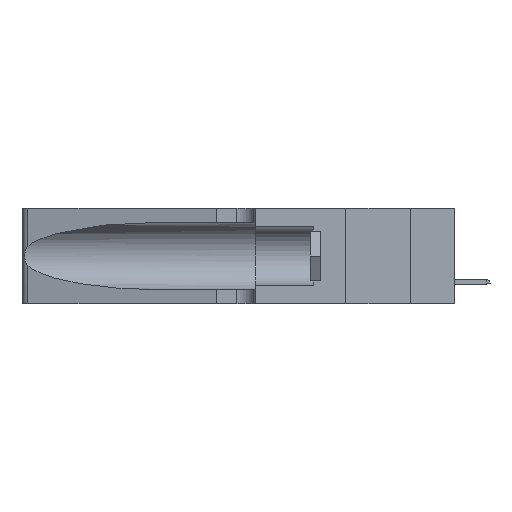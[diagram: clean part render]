
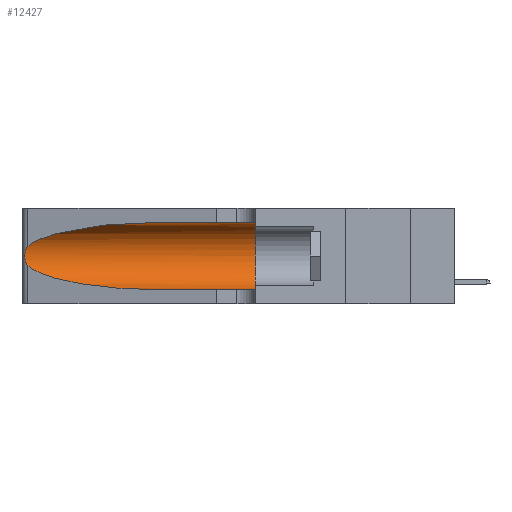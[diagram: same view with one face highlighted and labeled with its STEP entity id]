
A CAD part, left-side view. The second image highlights one B-rep face of the part: STEP entity #12427.
In plain terms, the highlighted cylindrical face has radius 3.308 mm (diameter 6.617 mm), a partial arc.
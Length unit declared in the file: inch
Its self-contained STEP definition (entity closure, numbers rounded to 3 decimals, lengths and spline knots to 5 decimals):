
#204 = CARTESIAN_POINT ( 'NONE',  ( 0.18966, 0.96281, 0.05475 ) ) ;
#894 = LINE ( 'NONE', #17572, #18752 ) ;
#1700 = EDGE_CURVE ( 'NONE', #21405, #21817, #20528, .T. ) ;
#2361 = CARTESIAN_POINT ( 'NONE',  ( 0.2373, 1.15595, 0.08982 ) ) ;
#3760 = CARTESIAN_POINT ( 'NONE',  ( 0.2373, 1.15595, 0.28018 ) ) ;
#3841 = CARTESIAN_POINT ( 'NONE',  ( 0.25787, 1.23484, 0.2124 ) ) ;
#4401 = CARTESIAN_POINT ( 'NONE',  ( 0.1305, 0.35, 0.185 ) ) ;
#4836 = ORIENTED_EDGE ( 'NONE', *, *, #15685, .T. ) ;
#4950 = FACE_OUTER_BOUND ( 'NONE', #5608, .T. ) ;
#5600 = CARTESIAN_POINT ( 'NONE',  ( 0.25854, 1.2359, 0.20912 ) ) ;
#5608 = EDGE_LOOP ( 'NONE', ( #13144, #4836, #24133, #20268, #17109, #25345 ) ) ;
#6421 = DIRECTION ( 'NONE',  ( 0., 1., 0. ) ) ;
#7059 = CARTESIAN_POINT ( 'NONE',  ( 0.1305, 0.35, 0.31525 ) ) ;
#7375 = EDGE_CURVE ( 'NONE', #21405, #19061, #19335, .T. ) ;
#7846 = CARTESIAN_POINT ( 'NONE',  ( 0.1305, 0.72297, 0.31525 ) ) ;
#7878 = CARTESIAN_POINT ( 'NONE',  ( 0.26075, 1.23896, 0.178 ) ) ;
#8137 = CARTESIAN_POINT ( 'NONE',  ( 0.25487, 1.22718, 0.14631 ) ) ;
#8306 = CARTESIAN_POINT ( 'NONE',  ( 0.1305, 0.72297, 0.05475 ) ) ;
#8757 = AXIS2_PLACEMENT_3D ( 'NONE', #4401, #6421, #14668 ) ;
#9777 = CARTESIAN_POINT ( 'NONE',  ( 0.25856, 1.23593, 0.16098 ) ) ;
#10253 = CYLINDRICAL_SURFACE ( 'NONE', #23731, 0.13025 ) ;
#10320 = VERTEX_POINT ( 'NONE', #11181 ) ;
#11181 = CARTESIAN_POINT ( 'NONE',  ( 0.1305, 0.72297, 0.05475 ) ) ;
#11293 = CARTESIAN_POINT ( 'NONE',  ( 0.25487, 1.22718, 0.22369 ) ) ;
#11304 = DIRECTION ( 'NONE',  ( 0., -1., 0. ) ) ;
#11709 = DIRECTION ( 'NONE',  ( 0., -1., 0. ) ) ;
#12253 = CARTESIAN_POINT ( 'NONE',  ( 0.25487, 1.22718, 0.22369 ) ) ;
#12276 = DIRECTION ( 'NONE',  ( 0., 0., -1. ) ) ;
#12427 = ADVANCED_FACE ( 'NONE', ( #4950 ), #10253, .F. ) ;
#13144 = ORIENTED_EDGE ( 'NONE', *, *, #1700, .T. ) ;
#13708 = CARTESIAN_POINT ( 'NONE',  ( 0.26018, 1.23835, 0.19895 ) ) ;
#13839 = CARTESIAN_POINT ( 'NONE',  ( 0.25789, 1.23486, 0.15765 ) ) ;
#14086 = EDGE_CURVE ( 'NONE', #10320, #23124, #894, .T. ) ;
#14668 = DIRECTION ( 'NONE',  ( 0., 0., 1. ) ) ;
#15224 = CARTESIAN_POINT ( 'NONE',  ( 0.1305, 1.61858, 0.31525 ) ) ;
#15685 = EDGE_CURVE ( 'NONE', #21817, #23894, #21483, .T. ) ;
#15830 = CARTESIAN_POINT ( 'NONE',  ( 0.25555, 1.22994, 0.2215 ) ) ;
#17109 = ORIENTED_EDGE ( 'NONE', *, *, #23506, .F. ) ;
#17188 = CARTESIAN_POINT ( 'NONE',  ( 0.1305, 0.35, 0.05475 ) ) ;
#17572 = CARTESIAN_POINT ( 'NONE',  ( 0.1305, 1.61858, 0.05475 ) ) ;
#17819 = CARTESIAN_POINT ( 'NONE',  ( 0.25639, 1.23186, 0.15144 ) ) ;
#17967 =( BOUNDED_CURVE ( )  B_SPLINE_CURVE ( 3, ( #24764, #2361, #204, #8306 ),
 .UNSPECIFIED., .F., .F. ) 
 B_SPLINE_CURVE_WITH_KNOTS ( ( 4, 4 ),
 ( 3.44316, 4.71239 ),
 .UNSPECIFIED. ) 
 CURVE ( )  GEOMETRIC_REPRESENTATION_ITEM ( )  RATIONAL_B_SPLINE_CURVE ( ( 1., 0.87, 0.87, 1. ) ) 
 REPRESENTATION_ITEM ( '' )  );
#18008 = CARTESIAN_POINT ( 'NONE',  ( 0.1305, 0.72297, 0.31525 ) ) ;
#18082 = CARTESIAN_POINT ( 'NONE',  ( 0.25639, 1.23184, 0.21858 ) ) ;
#18752 = VECTOR ( 'NONE', #11304, 39.37008 ) ;
#19061 = VERTEX_POINT ( 'NONE', #7059 ) ;
#19335 = LINE ( 'NONE', #15224, #23375 ) ;
#19949 = CARTESIAN_POINT ( 'NONE',  ( 0.25487, 1.22718, 0.22369 ) ) ;
#20268 = ORIENTED_EDGE ( 'NONE', *, *, #14086, .T. ) ;
#20528 =( BOUNDED_CURVE ( )  B_SPLINE_CURVE ( 3, ( #18008, #24125, #3760, #12253 ),
 .UNSPECIFIED., .F., .T. ) 
 B_SPLINE_CURVE_WITH_KNOTS ( ( 4, 4 ),
 ( 1.5708, 2.84003 ),
 .UNSPECIFIED. ) 
 CURVE ( )  GEOMETRIC_REPRESENTATION_ITEM ( )  RATIONAL_B_SPLINE_CURVE ( ( 1., 0.87, 0.87, 1. ) ) 
 REPRESENTATION_ITEM ( '' )  );
#21405 = VERTEX_POINT ( 'NONE', #7846 ) ;
#21483 = B_SPLINE_CURVE_WITH_KNOTS ( 'NONE', 3,
 ( #19949, #15830, #18082, #3841, #5600, #13708, #23940, #7878, #22037, #9777, #13839, #17819, #21914, #22167 ),
 .UNSPECIFIED., .F., .F.,
 ( 4, 2, 2, 2, 2, 2, 4 ),
 ( 0., 0.00027, 0.00053, 0.00107, 0.0016, 0.00187, 0.00214 ),
 .UNSPECIFIED. ) ;
#21817 = VERTEX_POINT ( 'NONE', #11293 ) ;
#21914 = CARTESIAN_POINT ( 'NONE',  ( 0.25555, 1.22993, 0.14849 ) ) ;
#22037 = CARTESIAN_POINT ( 'NONE',  ( 0.26017, 1.23833, 0.17102 ) ) ;
#22167 = CARTESIAN_POINT ( 'NONE',  ( 0.25487, 1.22718, 0.14631 ) ) ;
#22667 = CARTESIAN_POINT ( 'NONE',  ( 0.1305, 1.61858, 0.185 ) ) ;
#23124 = VERTEX_POINT ( 'NONE', #17188 ) ;
#23375 = VECTOR ( 'NONE', #11709, 39.37008 ) ;
#23506 = EDGE_CURVE ( 'NONE', #19061, #23124, #25405, .T. ) ;
#23731 = AXIS2_PLACEMENT_3D ( 'NONE', #22667, #24404, #12276 ) ;
#23894 = VERTEX_POINT ( 'NONE', #8137 ) ;
#23940 = CARTESIAN_POINT ( 'NONE',  ( 0.26075, 1.23896, 0.19203 ) ) ;
#24125 = CARTESIAN_POINT ( 'NONE',  ( 0.18966, 0.96281, 0.31525 ) ) ;
#24133 = ORIENTED_EDGE ( 'NONE', *, *, #26510, .T. ) ;
#24404 = DIRECTION ( 'NONE',  ( 0., -1., 0. ) ) ;
#24764 = CARTESIAN_POINT ( 'NONE',  ( 0.25487, 1.22718, 0.14631 ) ) ;
#25345 = ORIENTED_EDGE ( 'NONE', *, *, #7375, .F. ) ;
#25405 = CIRCLE ( 'NONE', #8757, 0.13025 ) ;
#26510 = EDGE_CURVE ( 'NONE', #23894, #10320, #17967, .T. ) ;
